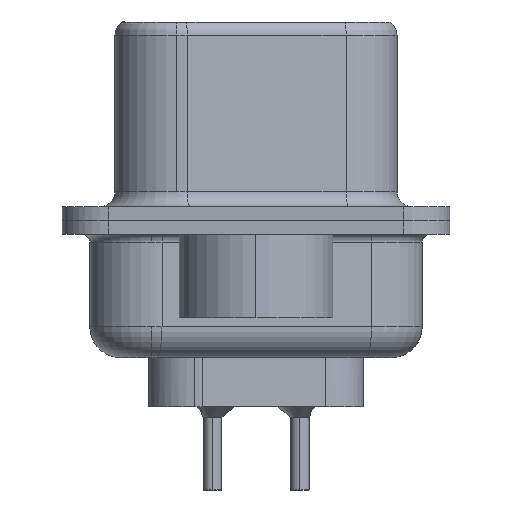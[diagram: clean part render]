
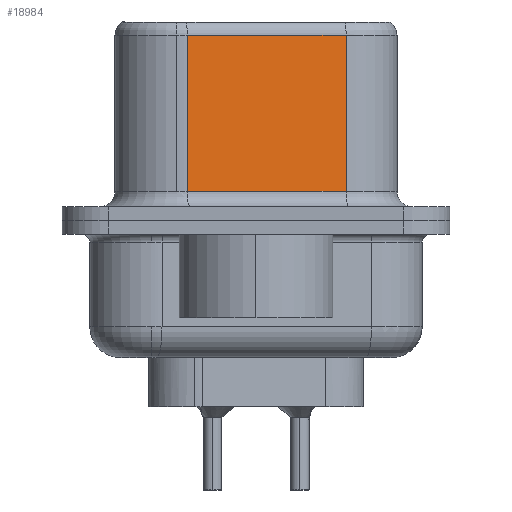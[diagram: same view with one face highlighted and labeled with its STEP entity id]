
A CAD part, left-side view. The second image highlights one B-rep face of the part: STEP entity #18984.
In plain terms, the highlighted planar face has unit normal (-0.985, -0.174, 0).
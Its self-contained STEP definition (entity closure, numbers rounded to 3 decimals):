
#1131 = CARTESIAN_POINT ( 'NONE',  ( 4.575, -2.927, 0.95 ) ) ;
#2706 = VECTOR ( 'NONE', #6003, 1000. ) ;
#3480 = LINE ( 'NONE', #14947, #11274 ) ;
#3970 = DIRECTION ( 'NONE',  ( 0., 0., -1. ) ) ;
#4008 = ORIENTED_EDGE ( 'NONE', *, *, #21231, .T. ) ;
#4558 = CARTESIAN_POINT ( 'NONE',  ( 4.575, -2.927, 0.95 ) ) ;
#5358 = AXIS2_PLACEMENT_3D ( 'NONE', #7436, #18847, #9071 ) ;
#5377 = CARTESIAN_POINT ( 'NONE',  ( 4.575, -2.927, 6.02 ) ) ;
#6003 = DIRECTION ( 'NONE',  ( -0.174, 0.985, 0. ) ) ;
#6024 = ORIENTED_EDGE ( 'NONE', *, *, #20961, .T. ) ;
#7436 = CARTESIAN_POINT ( 'NONE',  ( 4.575, -2.927, 6.52 ) ) ;
#8949 = ORIENTED_EDGE ( 'NONE', *, *, #21414, .F. ) ;
#9071 = DIRECTION ( 'NONE',  ( -0.174, 0.985, 0. ) ) ;
#11274 = VECTOR ( 'NONE', #16600, 1000. ) ;
#12038 = VECTOR ( 'NONE', #3970, 1000. ) ;
#12116 = LINE ( 'NONE', #4558, #13108 ) ;
#12187 = CARTESIAN_POINT ( 'NONE',  ( 3.665, 2.233, 0.95 ) ) ;
#13108 = VECTOR ( 'NONE', #14420, 1000. ) ;
#14420 = DIRECTION ( 'NONE',  ( 0.174, -0.985, 0. ) ) ;
#14947 = CARTESIAN_POINT ( 'NONE',  ( 3.665, 2.233, 6.52 ) ) ;
#15586 = PLANE ( 'NONE',  #5358 ) ;
#15915 = LINE ( 'NONE', #17471, #2706 ) ;
#16600 = DIRECTION ( 'NONE',  ( 0., 0., -1. ) ) ;
#16900 = LINE ( 'NONE', #17151, #12038 ) ;
#16995 = ORIENTED_EDGE ( 'NONE', *, *, #19230, .T. ) ;
#17151 = CARTESIAN_POINT ( 'NONE',  ( 4.575, -2.927, 6.52 ) ) ;
#17471 = CARTESIAN_POINT ( 'NONE',  ( 4.575, -2.927, 6.02 ) ) ;
#17617 = VERTEX_POINT ( 'NONE', #5377 ) ;
#17726 = VERTEX_POINT ( 'NONE', #12187 ) ;
#18311 = VERTEX_POINT ( 'NONE', #20478 ) ;
#18506 = VERTEX_POINT ( 'NONE', #1131 ) ;
#18847 = DIRECTION ( 'NONE',  ( 0.985, 0.174, 0. ) ) ;
#18984 = ADVANCED_FACE ( 'NONE', ( #20060 ), #15586, .F. ) ;
#19230 = EDGE_CURVE ( 'NONE', #17726, #18506, #12116, .T. ) ;
#20060 = FACE_OUTER_BOUND ( 'NONE', #20152, .T. ) ;
#20152 = EDGE_LOOP ( 'NONE', ( #8949, #6024, #4008, #16995 ) ) ;
#20478 = CARTESIAN_POINT ( 'NONE',  ( 3.665, 2.233, 6.02 ) ) ;
#20961 = EDGE_CURVE ( 'NONE', #17617, #18311, #15915, .T. ) ;
#21231 = EDGE_CURVE ( 'NONE', #18311, #17726, #3480, .T. ) ;
#21414 = EDGE_CURVE ( 'NONE', #17617, #18506, #16900, .T. ) ;
